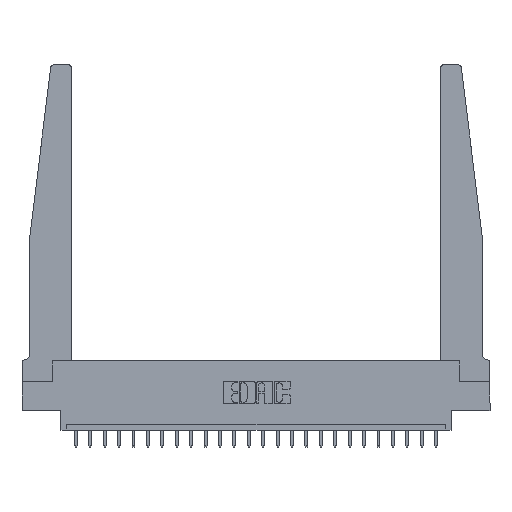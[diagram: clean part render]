
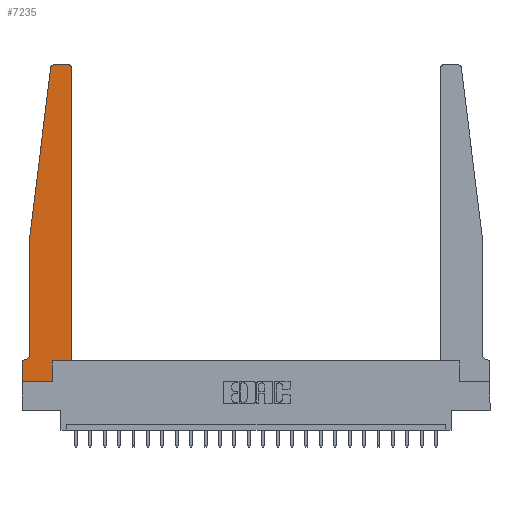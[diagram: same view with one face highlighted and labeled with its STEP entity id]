
A CAD part, top view. The second image highlights one B-rep face of the part: STEP entity #7235.
In plain terms, the highlighted planar face has unit normal (0, 0, 1).
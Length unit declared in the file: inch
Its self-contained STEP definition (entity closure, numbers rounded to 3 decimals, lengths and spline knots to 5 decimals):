
#150 = EDGE_CURVE ( 'NONE', #22889, #628, #15095, .T. ) ;
#446 = DIRECTION ( 'NONE',  ( 0., -1., 0. ) ) ;
#628 = VERTEX_POINT ( 'NONE', #3495 ) ;
#783 = DIRECTION ( 'NONE',  ( -0.122, -0.992, 0. ) ) ;
#841 = CARTESIAN_POINT ( 'NONE',  ( 0.2605, 0., 0.37 ) ) ;
#1002 = DIRECTION ( 'NONE',  ( 1., 0., 0. ) ) ;
#1410 = DIRECTION ( 'NONE',  ( 0., 1., 0. ) ) ;
#1447 = CARTESIAN_POINT ( 'NONE',  ( 0.395, 2.72, 0.37 ) ) ;
#1560 = VERTEX_POINT ( 'NONE', #17769 ) ;
#1763 = AXIS2_PLACEMENT_3D ( 'NONE', #5097, #12297, #19334 ) ;
#2403 = FACE_OUTER_BOUND ( 'NONE', #19680, .T. ) ;
#2407 = ORIENTED_EDGE ( 'NONE', *, *, #19723, .T. ) ;
#2508 = CARTESIAN_POINT ( 'NONE',  ( 0.065, 1.25, 0.37 ) ) ;
#3150 = CIRCLE ( 'NONE', #19884, 0.05 ) ;
#3331 = DIRECTION ( 'NONE',  ( 0., 0., 1. ) ) ;
#3397 = EDGE_CURVE ( 'NONE', #22404, #14085, #3150, .T. ) ;
#3495 = CARTESIAN_POINT ( 'NONE',  ( 0.2605, 0.18, 0.37 ) ) ;
#3582 = VECTOR ( 'NONE', #1410, 39.37008 ) ;
#3606 = VERTEX_POINT ( 'NONE', #6772 ) ;
#3618 = EDGE_CURVE ( 'NONE', #3606, #12445, #9618, .T. ) ;
#4000 = CARTESIAN_POINT ( 'NONE',  ( 0.425, 0.18, 0.37 ) ) ;
#4572 = EDGE_CURVE ( 'NONE', #4734, #19627, #6756, .T. ) ;
#4734 = VERTEX_POINT ( 'NONE', #11203 ) ;
#5097 = CARTESIAN_POINT ( 'NONE',  ( 0.27653, 2.72, 0.37 ) ) ;
#5200 = VECTOR ( 'NONE', #12506, 39.37008 ) ;
#5410 = DIRECTION ( 'NONE',  ( -1., 0., 0. ) ) ;
#5557 = VERTEX_POINT ( 'NONE', #7855 ) ;
#5638 = CARTESIAN_POINT ( 'NONE',  ( 0.25, 2.75, 0.37 ) ) ;
#5951 = CARTESIAN_POINT ( 'NONE',  ( 0.065, 1.25, 0.37 ) ) ;
#6234 = DIRECTION ( 'NONE',  ( 0., 0., 1. ) ) ;
#6254 = ORIENTED_EDGE ( 'NONE', *, *, #22427, .T. ) ;
#6320 = CARTESIAN_POINT ( 'NONE',  ( 0.015, 0.2375, 0.37 ) ) ;
#6756 = CIRCLE ( 'NONE', #1763, 0.03 ) ;
#6772 = CARTESIAN_POINT ( 'NONE',  ( 0., 0.1875, 0.37 ) ) ;
#6922 = AXIS2_PLACEMENT_3D ( 'NONE', #8685, #3331, #8772 ) ;
#7150 = EDGE_CURVE ( 'NONE', #5557, #13488, #16436, .T. ) ;
#7235 = ADVANCED_FACE ( 'NONE', ( #2403 ), #14227, .T. ) ;
#7638 = VECTOR ( 'NONE', #1002, 39.37008 ) ;
#7855 = CARTESIAN_POINT ( 'NONE',  ( 0.425, 2.72, 0.37 ) ) ;
#7953 = ORIENTED_EDGE ( 'NONE', *, *, #22727, .T. ) ;
#8033 = LINE ( 'NONE', #4000, #17815 ) ;
#8128 = EDGE_CURVE ( 'NONE', #14085, #3606, #13627, .T. ) ;
#8582 = CARTESIAN_POINT ( 'NONE',  ( 0.2605, 0.18, 0.37 ) ) ;
#8685 = CARTESIAN_POINT ( 'NONE',  ( 0., 0.1875, 0.37 ) ) ;
#8772 = DIRECTION ( 'NONE',  ( 1., 0., 0. ) ) ;
#9313 = ORIENTED_EDGE ( 'NONE', *, *, #15678, .T. ) ;
#9337 = ORIENTED_EDGE ( 'NONE', *, *, #3618, .T. ) ;
#9545 = EDGE_CURVE ( 'NONE', #628, #1560, #19667, .T. ) ;
#9618 = LINE ( 'NONE', #16233, #18264 ) ;
#9902 = VECTOR ( 'NONE', #5410, 39.37008 ) ;
#10016 = ORIENTED_EDGE ( 'NONE', *, *, #3397, .T. ) ;
#10269 = DIRECTION ( 'NONE',  ( 1., 0., 0. ) ) ;
#10528 = DIRECTION ( 'NONE',  ( 1., 0., 0. ) ) ;
#11203 = CARTESIAN_POINT ( 'NONE',  ( 0.27653, 2.75, 0.37 ) ) ;
#12097 = LINE ( 'NONE', #5951, #21598 ) ;
#12297 = DIRECTION ( 'NONE',  ( 0., 0., 1. ) ) ;
#12445 = VERTEX_POINT ( 'NONE', #20689 ) ;
#12506 = DIRECTION ( 'NONE',  ( -1., 0., 0. ) ) ;
#12742 = ORIENTED_EDGE ( 'NONE', *, *, #150, .T. ) ;
#12777 = DIRECTION ( 'NONE',  ( 0., 1., 0. ) ) ;
#13004 = LINE ( 'NONE', #21440, #23073 ) ;
#13218 = CARTESIAN_POINT ( 'NONE',  ( 0.015, 0.1875, 0.37 ) ) ;
#13488 = VERTEX_POINT ( 'NONE', #20700 ) ;
#13627 = LINE ( 'NONE', #19694, #5200 ) ;
#14085 = VERTEX_POINT ( 'NONE', #13218 ) ;
#14227 = PLANE ( 'NONE',  #6922 ) ;
#14261 = AXIS2_PLACEMENT_3D ( 'NONE', #1447, #6234, #10269 ) ;
#14353 = ORIENTED_EDGE ( 'NONE', *, *, #9545, .T. ) ;
#14732 = LINE ( 'NONE', #2508, #17524 ) ;
#15095 = LINE ( 'NONE', #8582, #3582 ) ;
#15678 = EDGE_CURVE ( 'NONE', #19627, #17697, #14732, .T. ) ;
#16233 = CARTESIAN_POINT ( 'NONE',  ( 0., 0., 0.37 ) ) ;
#16436 = CIRCLE ( 'NONE', #14261, 0.03 ) ;
#16618 = EDGE_CURVE ( 'NONE', #12445, #22889, #13004, .T. ) ;
#16880 = LINE ( 'NONE', #5638, #9902 ) ;
#17220 = CARTESIAN_POINT ( 'NONE',  ( 0.425, 0.18, 0.37 ) ) ;
#17524 = VECTOR ( 'NONE', #783, 39.37008 ) ;
#17647 = CARTESIAN_POINT ( 'NONE',  ( 0.24675, 2.72367, 0.37 ) ) ;
#17697 = VERTEX_POINT ( 'NONE', #22007 ) ;
#17769 = CARTESIAN_POINT ( 'NONE',  ( 0.425, 0.18, 0.37 ) ) ;
#17815 = VECTOR ( 'NONE', #12777, 39.37008 ) ;
#18197 = ORIENTED_EDGE ( 'NONE', *, *, #7150, .T. ) ;
#18212 = CARTESIAN_POINT ( 'NONE',  ( 0.065, 0.2375, 0.37 ) ) ;
#18264 = VECTOR ( 'NONE', #19668, 39.37008 ) ;
#19334 = DIRECTION ( 'NONE',  ( 1., 0., 0. ) ) ;
#19627 = VERTEX_POINT ( 'NONE', #17647 ) ;
#19667 = LINE ( 'NONE', #17220, #7638 ) ;
#19668 = DIRECTION ( 'NONE',  ( 0., -1., 0. ) ) ;
#19680 = EDGE_LOOP ( 'NONE', ( #6254, #21800, #9313, #7953, #10016, #22818, #9337, #21929, #12742, #14353, #2407, #18197 ) ) ;
#19694 = CARTESIAN_POINT ( 'NONE',  ( 0.065, 0.1875, 0.37 ) ) ;
#19723 = EDGE_CURVE ( 'NONE', #1560, #5557, #8033, .T. ) ;
#19884 = AXIS2_PLACEMENT_3D ( 'NONE', #6320, #22502, #20938 ) ;
#20689 = CARTESIAN_POINT ( 'NONE',  ( 0., 0., 0.37 ) ) ;
#20700 = CARTESIAN_POINT ( 'NONE',  ( 0.395, 2.75, 0.37 ) ) ;
#20938 = DIRECTION ( 'NONE',  ( -1., 0., 0. ) ) ;
#21440 = CARTESIAN_POINT ( 'NONE',  ( 0., 0., 0.37 ) ) ;
#21598 = VECTOR ( 'NONE', #446, 39.37008 ) ;
#21800 = ORIENTED_EDGE ( 'NONE', *, *, #4572, .T. ) ;
#21929 = ORIENTED_EDGE ( 'NONE', *, *, #16618, .T. ) ;
#22007 = CARTESIAN_POINT ( 'NONE',  ( 0.065, 1.25, 0.37 ) ) ;
#22404 = VERTEX_POINT ( 'NONE', #18212 ) ;
#22427 = EDGE_CURVE ( 'NONE', #13488, #4734, #16880, .T. ) ;
#22502 = DIRECTION ( 'NONE',  ( 0., 0., -1. ) ) ;
#22727 = EDGE_CURVE ( 'NONE', #17697, #22404, #12097, .T. ) ;
#22818 = ORIENTED_EDGE ( 'NONE', *, *, #8128, .T. ) ;
#22889 = VERTEX_POINT ( 'NONE', #841 ) ;
#23073 = VECTOR ( 'NONE', #10528, 39.37008 ) ;
